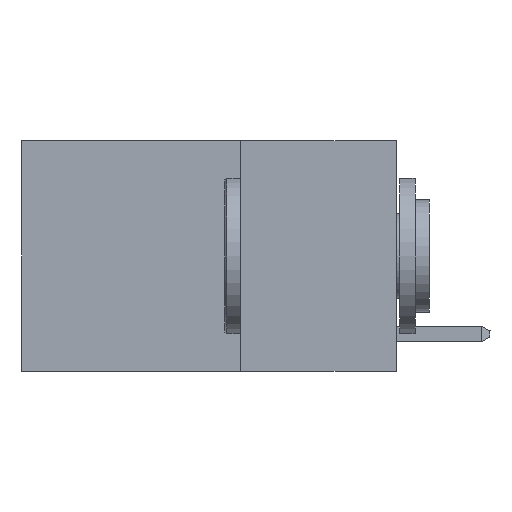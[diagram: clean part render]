
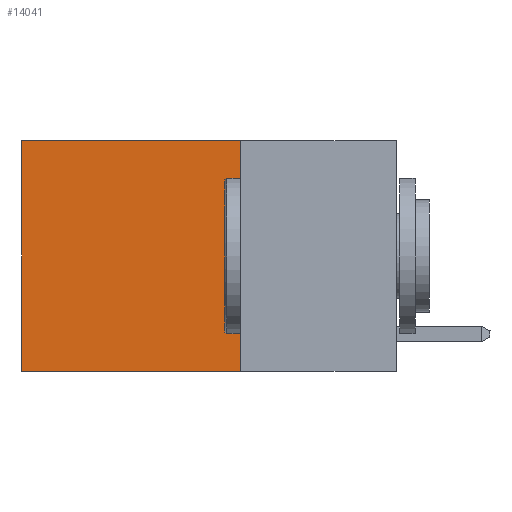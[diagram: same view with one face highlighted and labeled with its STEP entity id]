
A CAD part, left-side view. The second image highlights one B-rep face of the part: STEP entity #14041.
In plain terms, the highlighted planar face has unit normal (-1, 0, 0).
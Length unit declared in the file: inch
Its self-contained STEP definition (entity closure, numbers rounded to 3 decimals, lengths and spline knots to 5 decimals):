
#606 = CARTESIAN_POINT ( 'NONE',  ( 0.2625, 0.25, 0. ) ) ;
#723 = CARTESIAN_POINT ( 'NONE',  ( 0.2625, 0.25, -0.37 ) ) ;
#2807 = LINE ( 'NONE', #5404, #17578 ) ;
#3207 = CARTESIAN_POINT ( 'NONE',  ( 0.2625, 0.25, 0. ) ) ;
#3868 = EDGE_CURVE ( 'NONE', #18634, #22105, #26252, .T. ) ;
#4854 = VECTOR ( 'NONE', #24265, 39.37008 ) ;
#5225 = VERTEX_POINT ( 'NONE', #3207 ) ;
#5348 = CARTESIAN_POINT ( 'NONE',  ( 0.2625, 0.6, 0. ) ) ;
#5404 = CARTESIAN_POINT ( 'NONE',  ( 0.2625, 0.25, 0. ) ) ;
#6696 = PLANE ( 'NONE',  #17170 ) ;
#6763 = LINE ( 'NONE', #8944, #28102 ) ;
#6837 = CARTESIAN_POINT ( 'NONE',  ( 0.2625, 0.6, -0.37 ) ) ;
#7157 = DIRECTION ( 'NONE',  ( 1., 0., 0. ) ) ;
#8944 = CARTESIAN_POINT ( 'NONE',  ( 0.2625, 0.25, -0.37 ) ) ;
#10770 = EDGE_LOOP ( 'NONE', ( #26870, #23679, #14168, #22873 ) ) ;
#13770 = VERTEX_POINT ( 'NONE', #723 ) ;
#14041 = ADVANCED_FACE ( 'NONE', ( #21120 ), #6696, .F. ) ;
#14168 = ORIENTED_EDGE ( 'NONE', *, *, #24554, .F. ) ;
#16055 = VECTOR ( 'NONE', #21475, 39.37008 ) ;
#16466 = CARTESIAN_POINT ( 'NONE',  ( 0.2625, 0.25, 0. ) ) ;
#17170 = AXIS2_PLACEMENT_3D ( 'NONE', #16466, #7157, #30412 ) ;
#17578 = VECTOR ( 'NONE', #26153, 39.37008 ) ;
#18634 = VERTEX_POINT ( 'NONE', #28914 ) ;
#21120 = FACE_OUTER_BOUND ( 'NONE', #10770, .T. ) ;
#21475 = DIRECTION ( 'NONE',  ( 0., 0., -1. ) ) ;
#21803 = LINE ( 'NONE', #606, #4854 ) ;
#22105 = VERTEX_POINT ( 'NONE', #6837 ) ;
#22814 = EDGE_CURVE ( 'NONE', #13770, #22105, #6763, .T. ) ;
#22873 = ORIENTED_EDGE ( 'NONE', *, *, #26364, .T. ) ;
#23679 = ORIENTED_EDGE ( 'NONE', *, *, #22814, .F. ) ;
#24265 = DIRECTION ( 'NONE',  ( 0., 1., 0. ) ) ;
#24554 = EDGE_CURVE ( 'NONE', #5225, #13770, #2807, .T. ) ;
#25655 = DIRECTION ( 'NONE',  ( 0., 1., 0. ) ) ;
#26153 = DIRECTION ( 'NONE',  ( 0., 0., -1. ) ) ;
#26252 = LINE ( 'NONE', #5348, #16055 ) ;
#26364 = EDGE_CURVE ( 'NONE', #5225, #18634, #21803, .T. ) ;
#26870 = ORIENTED_EDGE ( 'NONE', *, *, #3868, .T. ) ;
#28102 = VECTOR ( 'NONE', #25655, 39.37008 ) ;
#28914 = CARTESIAN_POINT ( 'NONE',  ( 0.2625, 0.6, 0. ) ) ;
#30412 = DIRECTION ( 'NONE',  ( 0., 0., -1. ) ) ;
